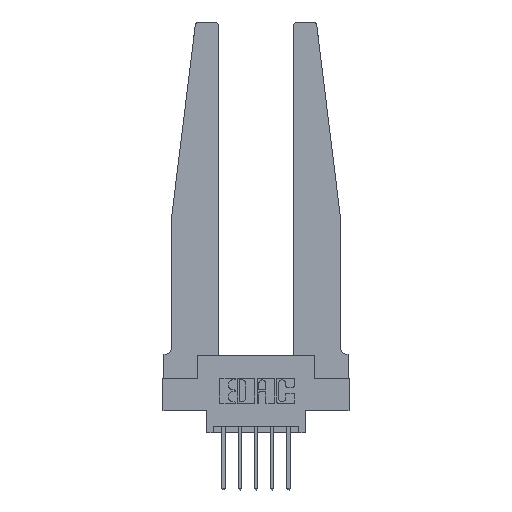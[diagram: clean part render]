
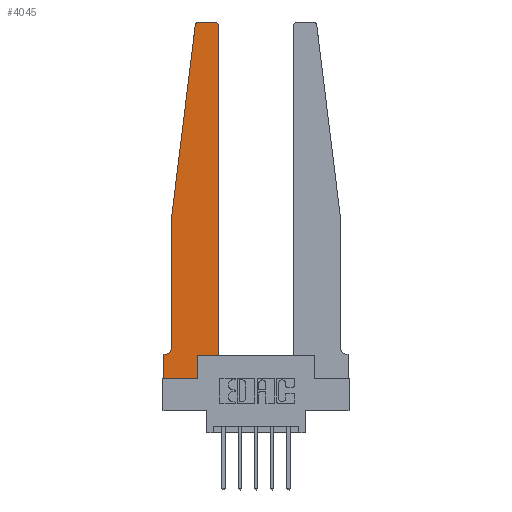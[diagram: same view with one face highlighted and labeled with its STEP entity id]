
A CAD part, top view. The second image highlights one B-rep face of the part: STEP entity #4045.
In plain terms, the highlighted planar face has unit normal (0, 0, 1).
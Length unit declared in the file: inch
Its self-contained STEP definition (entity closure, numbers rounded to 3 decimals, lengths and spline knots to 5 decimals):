
#521 = DIRECTION ( 'NONE',  ( 1., 0., 0. ) ) ;
#621 = VERTEX_POINT ( 'NONE', #1286 ) ;
#710 = VERTEX_POINT ( 'NONE', #11470 ) ;
#761 = LINE ( 'NONE', #13355, #9583 ) ;
#861 = CARTESIAN_POINT ( 'NONE',  ( 0.015, 0.2375, 0.37 ) ) ;
#874 = VECTOR ( 'NONE', #8249, 39.37008 ) ;
#942 = ORIENTED_EDGE ( 'NONE', *, *, #12272, .T. ) ;
#1049 = CARTESIAN_POINT ( 'NONE',  ( 0., 0.1875, 0.37 ) ) ;
#1250 = CARTESIAN_POINT ( 'NONE',  ( 0.065, 1.25, 0.37 ) ) ;
#1286 = CARTESIAN_POINT ( 'NONE',  ( 0.425, 2.72, 0.37 ) ) ;
#1341 = AXIS2_PLACEMENT_3D ( 'NONE', #11523, #2109, #11453 ) ;
#1487 = VECTOR ( 'NONE', #5460, 39.37008 ) ;
#1660 = VERTEX_POINT ( 'NONE', #6985 ) ;
#1757 = ORIENTED_EDGE ( 'NONE', *, *, #10502, .T. ) ;
#1815 = VERTEX_POINT ( 'NONE', #4285 ) ;
#1850 = LINE ( 'NONE', #3089, #874 ) ;
#1880 = VERTEX_POINT ( 'NONE', #1049 ) ;
#2092 = LINE ( 'NONE', #1250, #1487 ) ;
#2109 = DIRECTION ( 'NONE',  ( 0., 0., 1. ) ) ;
#2368 = ORIENTED_EDGE ( 'NONE', *, *, #4592, .T. ) ;
#2373 = DIRECTION ( 'NONE',  ( 0., 0., 1. ) ) ;
#2564 = VECTOR ( 'NONE', #521, 39.37008 ) ;
#2715 = CARTESIAN_POINT ( 'NONE',  ( 0.2605, 0.18, 0.37 ) ) ;
#2769 = VERTEX_POINT ( 'NONE', #13369 ) ;
#3089 = CARTESIAN_POINT ( 'NONE',  ( 0.065, 1.25, 0.37 ) ) ;
#3257 = VERTEX_POINT ( 'NONE', #12801 ) ;
#3809 = CARTESIAN_POINT ( 'NONE',  ( 0.425, 0.18, 0.37 ) ) ;
#3842 = AXIS2_PLACEMENT_3D ( 'NONE', #3922, #6285, #5104 ) ;
#3919 = CARTESIAN_POINT ( 'NONE',  ( 0.425, 0.18, 0.37 ) ) ;
#3922 = CARTESIAN_POINT ( 'NONE',  ( 0.27653, 2.72, 0.37 ) ) ;
#3989 = EDGE_CURVE ( 'NONE', #710, #1660, #5311, .T. ) ;
#4045 = ADVANCED_FACE ( 'NONE', ( #5536 ), #11779, .T. ) ;
#4096 = ORIENTED_EDGE ( 'NONE', *, *, #5131, .T. ) ;
#4285 = CARTESIAN_POINT ( 'NONE',  ( 0.24675, 2.72367, 0.37 ) ) ;
#4323 = EDGE_CURVE ( 'NONE', #10778, #621, #5099, .T. ) ;
#4430 = EDGE_CURVE ( 'NONE', #1880, #2769, #761, .T. ) ;
#4521 = CARTESIAN_POINT ( 'NONE',  ( 0.27653, 2.75, 0.37 ) ) ;
#4570 = DIRECTION ( 'NONE',  ( -1., 0., 0. ) ) ;
#4592 = EDGE_CURVE ( 'NONE', #12491, #10778, #7717, .T. ) ;
#4618 = LINE ( 'NONE', #8825, #7365 ) ;
#4939 = EDGE_CURVE ( 'NONE', #2769, #9252, #4618, .T. ) ;
#5063 = CARTESIAN_POINT ( 'NONE',  ( 0., 0.1875, 0.37 ) ) ;
#5099 = LINE ( 'NONE', #3919, #6271 ) ;
#5104 = DIRECTION ( 'NONE',  ( 1., 0., 0. ) ) ;
#5131 = EDGE_CURVE ( 'NONE', #5660, #1815, #6507, .T. ) ;
#5205 = ORIENTED_EDGE ( 'NONE', *, *, #3989, .T. ) ;
#5311 = CIRCLE ( 'NONE', #12563, 0.05 ) ;
#5460 = DIRECTION ( 'NONE',  ( -0.122, -0.992, 0. ) ) ;
#5465 = VECTOR ( 'NONE', #4570, 39.37008 ) ;
#5536 = FACE_OUTER_BOUND ( 'NONE', #13531, .T. ) ;
#5660 = VERTEX_POINT ( 'NONE', #4521 ) ;
#5677 = ORIENTED_EDGE ( 'NONE', *, *, #8041, .T. ) ;
#6167 = ORIENTED_EDGE ( 'NONE', *, *, #6734, .T. ) ;
#6271 = VECTOR ( 'NONE', #12453, 39.37008 ) ;
#6285 = DIRECTION ( 'NONE',  ( 0., 0., 1. ) ) ;
#6398 = ORIENTED_EDGE ( 'NONE', *, *, #7319, .T. ) ;
#6507 = CIRCLE ( 'NONE', #3842, 0.03 ) ;
#6734 = EDGE_CURVE ( 'NONE', #1660, #1880, #12367, .T. ) ;
#6752 = VERTEX_POINT ( 'NONE', #9302 ) ;
#6795 = ORIENTED_EDGE ( 'NONE', *, *, #4323, .T. ) ;
#6985 = CARTESIAN_POINT ( 'NONE',  ( 0.015, 0.1875, 0.37 ) ) ;
#7276 = CIRCLE ( 'NONE', #1341, 0.03 ) ;
#7319 = EDGE_CURVE ( 'NONE', #3257, #5660, #12130, .T. ) ;
#7365 = VECTOR ( 'NONE', #11161, 39.37008 ) ;
#7608 = DIRECTION ( 'NONE',  ( 0., 0., -1. ) ) ;
#7717 = LINE ( 'NONE', #9701, #2564 ) ;
#7756 = ORIENTED_EDGE ( 'NONE', *, *, #11760, .T. ) ;
#8041 = EDGE_CURVE ( 'NONE', #1815, #6752, #2092, .T. ) ;
#8249 = DIRECTION ( 'NONE',  ( 0., -1., 0. ) ) ;
#8557 = DIRECTION ( 'NONE',  ( -1., 0., 0. ) ) ;
#8825 = CARTESIAN_POINT ( 'NONE',  ( 0., 0., 0.37 ) ) ;
#9252 = VERTEX_POINT ( 'NONE', #11669 ) ;
#9291 = DIRECTION ( 'NONE',  ( 0., 1., 0. ) ) ;
#9302 = CARTESIAN_POINT ( 'NONE',  ( 0.065, 1.25, 0.37 ) ) ;
#9493 = CARTESIAN_POINT ( 'NONE',  ( 0.2605, 0.18, 0.37 ) ) ;
#9583 = VECTOR ( 'NONE', #10262, 39.37008 ) ;
#9701 = CARTESIAN_POINT ( 'NONE',  ( 0.425, 0.18, 0.37 ) ) ;
#9734 = DIRECTION ( 'NONE',  ( 1., 0., 0. ) ) ;
#10262 = DIRECTION ( 'NONE',  ( 0., -1., 0. ) ) ;
#10314 = VECTOR ( 'NONE', #11217, 39.37008 ) ;
#10502 = EDGE_CURVE ( 'NONE', #6752, #710, #1850, .T. ) ;
#10609 = AXIS2_PLACEMENT_3D ( 'NONE', #5063, #2373, #9734 ) ;
#10778 = VERTEX_POINT ( 'NONE', #3809 ) ;
#11010 = ORIENTED_EDGE ( 'NONE', *, *, #4430, .T. ) ;
#11161 = DIRECTION ( 'NONE',  ( 1., 0., 0. ) ) ;
#11217 = DIRECTION ( 'NONE',  ( -1., 0., 0. ) ) ;
#11287 = CARTESIAN_POINT ( 'NONE',  ( 0.065, 0.1875, 0.37 ) ) ;
#11453 = DIRECTION ( 'NONE',  ( 1., 0., 0. ) ) ;
#11470 = CARTESIAN_POINT ( 'NONE',  ( 0.065, 0.2375, 0.37 ) ) ;
#11523 = CARTESIAN_POINT ( 'NONE',  ( 0.395, 2.72, 0.37 ) ) ;
#11669 = CARTESIAN_POINT ( 'NONE',  ( 0.2605, 0., 0.37 ) ) ;
#11760 = EDGE_CURVE ( 'NONE', #9252, #12491, #12577, .T. ) ;
#11779 = PLANE ( 'NONE',  #10609 ) ;
#12130 = LINE ( 'NONE', #13106, #5465 ) ;
#12272 = EDGE_CURVE ( 'NONE', #621, #3257, #7276, .T. ) ;
#12367 = LINE ( 'NONE', #11287, #10314 ) ;
#12453 = DIRECTION ( 'NONE',  ( 0., 1., 0. ) ) ;
#12491 = VERTEX_POINT ( 'NONE', #2715 ) ;
#12563 = AXIS2_PLACEMENT_3D ( 'NONE', #861, #7608, #8557 ) ;
#12577 = LINE ( 'NONE', #9493, #13431 ) ;
#12649 = ORIENTED_EDGE ( 'NONE', *, *, #4939, .T. ) ;
#12801 = CARTESIAN_POINT ( 'NONE',  ( 0.395, 2.75, 0.37 ) ) ;
#13106 = CARTESIAN_POINT ( 'NONE',  ( 0.25, 2.75, 0.37 ) ) ;
#13355 = CARTESIAN_POINT ( 'NONE',  ( 0., 0., 0.37 ) ) ;
#13369 = CARTESIAN_POINT ( 'NONE',  ( 0., 0., 0.37 ) ) ;
#13431 = VECTOR ( 'NONE', #9291, 39.37008 ) ;
#13531 = EDGE_LOOP ( 'NONE', ( #6398, #4096, #5677, #1757, #5205, #6167, #11010, #12649, #7756, #2368, #6795, #942 ) ) ;
